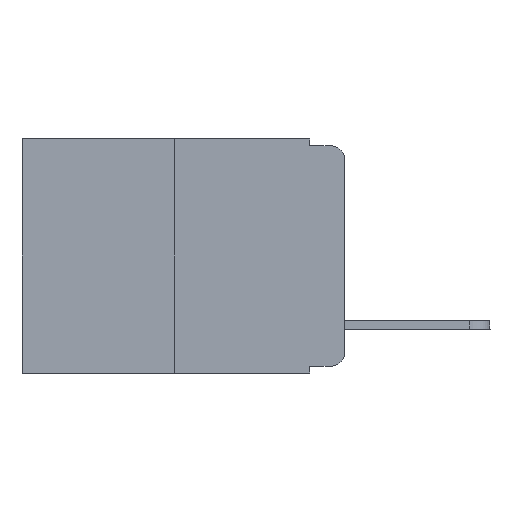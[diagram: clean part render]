
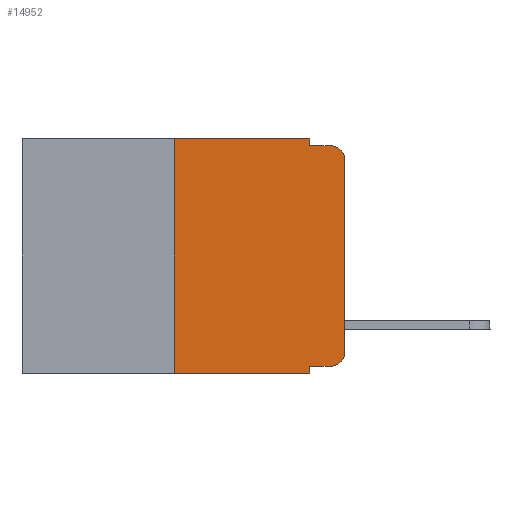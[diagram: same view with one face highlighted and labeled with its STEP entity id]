
A CAD part, left-side view. The second image highlights one B-rep face of the part: STEP entity #14952.
In plain terms, the highlighted planar face has unit normal (-1, 0, 0).
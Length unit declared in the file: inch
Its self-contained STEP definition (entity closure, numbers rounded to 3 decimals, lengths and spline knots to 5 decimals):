
#414 = CARTESIAN_POINT ( 'NONE',  ( 0., 0.473, 0. ) ) ;
#483 = EDGE_CURVE ( 'NONE', #18956, #16065, #6193, .T. ) ;
#1030 = EDGE_CURVE ( 'NONE', #5115, #7592, #4570, .T. ) ;
#1118 = EDGE_CURVE ( 'NONE', #9066, #6409, #16663, .T. ) ;
#1422 = VERTEX_POINT ( 'NONE', #11260 ) ;
#1447 = VECTOR ( 'NONE', #8872, 39.37008 ) ;
#1607 = CARTESIAN_POINT ( 'NONE',  ( 0., 0.473, 0. ) ) ;
#1694 = PLANE ( 'NONE',  #4672 ) ;
#2880 = DIRECTION ( 'NONE',  ( 0., -1., 0. ) ) ;
#2941 = DIRECTION ( 'NONE',  ( 0., -1., 0. ) ) ;
#3186 = CARTESIAN_POINT ( 'NONE',  ( 0., 0.051, -0.333 ) ) ;
#3522 = DIRECTION ( 'NONE',  ( 1., 0., 0. ) ) ;
#3556 = VERTEX_POINT ( 'NONE', #17081 ) ;
#3919 = EDGE_CURVE ( 'NONE', #6409, #1422, #20280, .T. ) ;
#4429 = CARTESIAN_POINT ( 'NONE',  ( 0., 0.25, -0.343 ) ) ;
#4570 = LINE ( 'NONE', #11078, #18238 ) ;
#4672 = AXIS2_PLACEMENT_3D ( 'NONE', #414, #3522, #5457 ) ;
#5072 = EDGE_CURVE ( 'NONE', #7592, #9066, #15120, .T. ) ;
#5115 = VERTEX_POINT ( 'NONE', #3186 ) ;
#5207 = DIRECTION ( 'NONE',  ( 0., 0., -1. ) ) ;
#5229 = CARTESIAN_POINT ( 'NONE',  ( 0., 0., 0. ) ) ;
#5277 = ORIENTED_EDGE ( 'NONE', *, *, #3919, .T. ) ;
#5457 = DIRECTION ( 'NONE',  ( 0., 0., -1. ) ) ;
#5484 = ORIENTED_EDGE ( 'NONE', *, *, #5072, .T. ) ;
#5552 = ORIENTED_EDGE ( 'NONE', *, *, #20903, .F. ) ;
#5816 = CARTESIAN_POINT ( 'NONE',  ( 0., 0.02, -0.333 ) ) ;
#6193 = LINE ( 'NONE', #1607, #14682 ) ;
#6291 = CARTESIAN_POINT ( 'NONE',  ( 0., 0.02, -0.313 ) ) ;
#6401 = EDGE_CURVE ( 'NONE', #3556, #1422, #19117, .T. ) ;
#6409 = VERTEX_POINT ( 'NONE', #14383 ) ;
#6615 = EDGE_LOOP ( 'NONE', ( #13004, #5277, #10937, #10205, #6988, #16457, #12539, #5552, #12802, #5484 ) ) ;
#6740 = DIRECTION ( 'NONE',  ( 0., 0., -1. ) ) ;
#6988 = ORIENTED_EDGE ( 'NONE', *, *, #483, .F. ) ;
#7418 = DIRECTION ( 'NONE',  ( 0., 0., 1. ) ) ;
#7592 = VERTEX_POINT ( 'NONE', #5816 ) ;
#7923 = AXIS2_PLACEMENT_3D ( 'NONE', #6291, #9465, #14287 ) ;
#8872 = DIRECTION ( 'NONE',  ( 0., 0., -1. ) ) ;
#8954 = EDGE_CURVE ( 'NONE', #16065, #3556, #15322, .T. ) ;
#9066 = VERTEX_POINT ( 'NONE', #12704 ) ;
#9465 = DIRECTION ( 'NONE',  ( -1., 0., 0. ) ) ;
#9816 = CARTESIAN_POINT ( 'NONE',  ( 0., 0.25, 0. ) ) ;
#9917 = LINE ( 'NONE', #14720, #11416 ) ;
#10205 = ORIENTED_EDGE ( 'NONE', *, *, #8954, .F. ) ;
#10937 = ORIENTED_EDGE ( 'NONE', *, *, #6401, .F. ) ;
#10973 = CARTESIAN_POINT ( 'NONE',  ( 0., 0.051, -0.01 ) ) ;
#11078 = CARTESIAN_POINT ( 'NONE',  ( 0., 0.051, -0.333 ) ) ;
#11260 = CARTESIAN_POINT ( 'NONE',  ( 0., 0.02, -0.01 ) ) ;
#11416 = VECTOR ( 'NONE', #6740, 39.37008 ) ;
#11480 = VERTEX_POINT ( 'NONE', #4429 ) ;
#11499 = EDGE_CURVE ( 'NONE', #11480, #16151, #15754, .T. ) ;
#12127 = DIRECTION ( 'NONE',  ( -1., 0., 0. ) ) ;
#12539 = ORIENTED_EDGE ( 'NONE', *, *, #11499, .T. ) ;
#12704 = CARTESIAN_POINT ( 'NONE',  ( 0., 0., -0.313 ) ) ;
#12802 = ORIENTED_EDGE ( 'NONE', *, *, #1030, .T. ) ;
#13004 = ORIENTED_EDGE ( 'NONE', *, *, #1118, .T. ) ;
#13809 = VECTOR ( 'NONE', #14695, 39.37008 ) ;
#14002 = CARTESIAN_POINT ( 'NONE',  ( 0., 0.051, -0.343 ) ) ;
#14287 = DIRECTION ( 'NONE',  ( 0., 0., -1. ) ) ;
#14383 = CARTESIAN_POINT ( 'NONE',  ( 0., 0., -0.03 ) ) ;
#14682 = VECTOR ( 'NONE', #20726, 39.37008 ) ;
#14695 = DIRECTION ( 'NONE',  ( 0., 0., 1. ) ) ;
#14720 = CARTESIAN_POINT ( 'NONE',  ( 0., 0.051, 0. ) ) ;
#14788 = VECTOR ( 'NONE', #2941, 39.37008 ) ;
#14952 = ADVANCED_FACE ( 'NONE', ( #20076 ), #1694, .F. ) ;
#15120 = CIRCLE ( 'NONE', #7923, 0.02 ) ;
#15322 = LINE ( 'NONE', #15537, #1447 ) ;
#15537 = CARTESIAN_POINT ( 'NONE',  ( 0., 0.051, 0. ) ) ;
#15554 = LINE ( 'NONE', #17359, #18029 ) ;
#15754 = LINE ( 'NONE', #20761, #14788 ) ;
#16065 = VERTEX_POINT ( 'NONE', #18932 ) ;
#16151 = VERTEX_POINT ( 'NONE', #14002 ) ;
#16457 = ORIENTED_EDGE ( 'NONE', *, *, #17024, .F. ) ;
#16663 = LINE ( 'NONE', #5229, #13809 ) ;
#17024 = EDGE_CURVE ( 'NONE', #11480, #18956, #15554, .T. ) ;
#17081 = CARTESIAN_POINT ( 'NONE',  ( 0., 0.051, -0.01 ) ) ;
#17359 = CARTESIAN_POINT ( 'NONE',  ( 0., 0.25, 0. ) ) ;
#17623 = DIRECTION ( 'NONE',  ( 0., -1., 0. ) ) ;
#18029 = VECTOR ( 'NONE', #7418, 39.37008 ) ;
#18238 = VECTOR ( 'NONE', #17623, 39.37008 ) ;
#18243 = CARTESIAN_POINT ( 'NONE',  ( 0., 0.02, -0.03 ) ) ;
#18932 = CARTESIAN_POINT ( 'NONE',  ( 0., 0.051, 0. ) ) ;
#18956 = VERTEX_POINT ( 'NONE', #9816 ) ;
#19117 = LINE ( 'NONE', #10973, #20297 ) ;
#19608 = AXIS2_PLACEMENT_3D ( 'NONE', #18243, #12127, #5207 ) ;
#20076 = FACE_OUTER_BOUND ( 'NONE', #6615, .T. ) ;
#20280 = CIRCLE ( 'NONE', #19608, 0.02 ) ;
#20297 = VECTOR ( 'NONE', #2880, 39.37008 ) ;
#20726 = DIRECTION ( 'NONE',  ( 0., -1., 0. ) ) ;
#20761 = CARTESIAN_POINT ( 'NONE',  ( 0., 0.473, -0.343 ) ) ;
#20903 = EDGE_CURVE ( 'NONE', #5115, #16151, #9917, .T. ) ;
